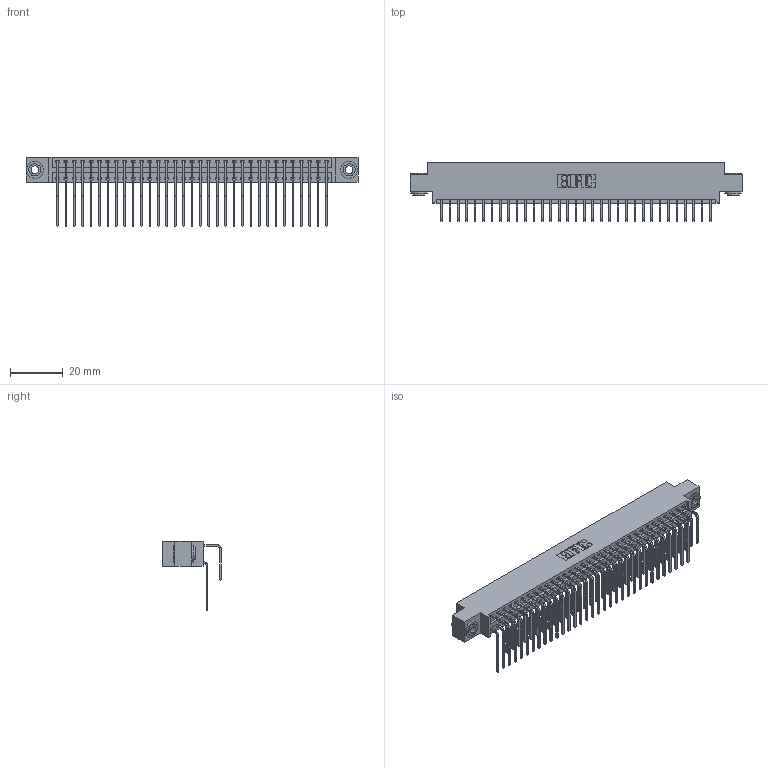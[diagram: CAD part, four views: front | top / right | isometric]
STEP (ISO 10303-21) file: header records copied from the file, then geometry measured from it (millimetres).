
FILE_DESCRIPTION (( 'STEP AP203' ), '1' );
FILE_NAME ('346-066-558-803.STEP', '2022-05-24T17:58:58', ( '' ), ( '' ), 'SwSTEP 2.0', 'SolidWorks 2020', '' );
FILE_SCHEMA (( 'CONFIG_CONTROL_DESIGN' ));
Length unit declared in the file: inch
Products named in the file (5): 345-292-001_558 Tail - 2; 345-292-001_558 559 Tail - 1; 346 Part_0.170 Offset - 0.156 Dia-TH; 345-250-002_345-250-002-102; 346-066-558-803
Assembly tree (69 placements, depth 2):
  346-066-558-803
    346 Part_0.170 Offset - 0.156 Dia-TH
    345-292-001_558 559 Tail - 1  x33
    345-292-001_558 Tail - 2  x33
    345-250-002_345-250-002-102  x2
Bounding box: 125.35 x 22.16 x 26.16 mm (x, y, z)
Volume: 12380.6 mm3; surface area: 19131.4 mm2
Topology: 69 solids, 69 shells, 3742 faces, 11079 edges, 7294 vertices
Faces by surface type: plane 2546, cylinder 1188, cone 8
Entity records: 25730 total; most frequent: CARTESIAN_POINT 4288, ORIENTED_EDGE 4162, DIRECTION 3831, EDGE_CURVE 2081, LINE 1753, VECTOR 1753, VERTEX_POINT 1382, AXIS2_PLACEMENT_3D 1039
